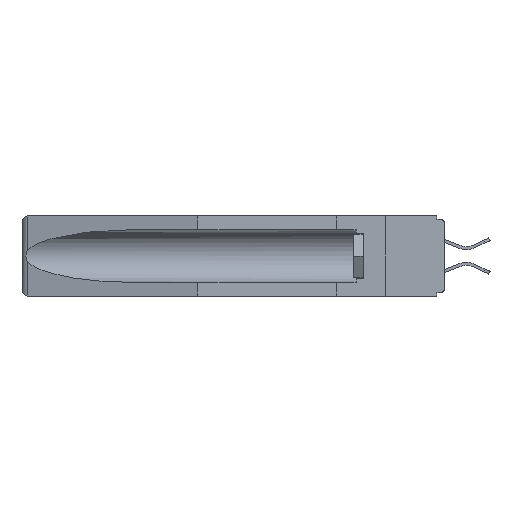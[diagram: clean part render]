
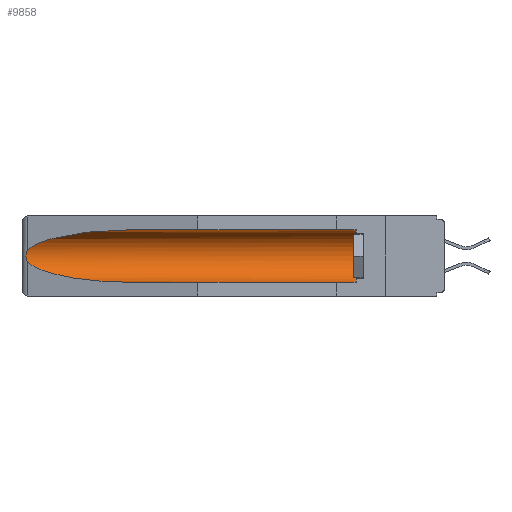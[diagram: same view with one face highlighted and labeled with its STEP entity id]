
A CAD part, left-side view. The second image highlights one B-rep face of the part: STEP entity #9858.
In plain terms, the highlighted cylindrical face has radius 2.857 mm (diameter 5.715 mm), a partial arc.
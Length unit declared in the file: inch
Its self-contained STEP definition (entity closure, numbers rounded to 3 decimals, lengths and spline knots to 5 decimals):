
#832 = CARTESIAN_POINT ( 'NONE',  ( 0.21114, 1.30732, -0.059 ) ) ;
#970 = EDGE_CURVE ( 'NONE', #17603, #32827, #12499, .T. ) ;
#3449 = VECTOR ( 'NONE', #21582, 39.37008 ) ;
#4038 = CARTESIAN_POINT ( 'NONE',  ( 0.2675, 1.53308, -0.16763 ) ) ;
#4170 = VERTEX_POINT ( 'NONE', #8145 ) ;
#4798 = CARTESIAN_POINT ( 'NONE',  ( 0.155, 1.07973, -0.059 ) ) ;
#6638 = ORIENTED_EDGE ( 'NONE', *, *, #20950, .T. ) ;
#6964 = FACE_OUTER_BOUND ( 'NONE', #16419, .T. ) ;
#7019 = CARTESIAN_POINT ( 'NONE',  ( 0.2673, 1.5327, -0.16383 ) ) ;
#7035 = CARTESIAN_POINT ( 'NONE',  ( 0.155, -0.30754, -0.284 ) ) ;
#7382 = CIRCLE ( 'NONE', #21650, 0.1125 ) ;
#7464 = CARTESIAN_POINT ( 'NONE',  ( 0.25451, 1.48313, -0.24835 ) ) ;
#7613 = ORIENTED_EDGE ( 'NONE', *, *, #23515, .T. ) ;
#8114 = DIRECTION ( 'NONE',  ( 0., 1., 0. ) ) ;
#8145 = CARTESIAN_POINT ( 'NONE',  ( 0.26537, 1.52718, -0.14972 ) ) ;
#8157 = ORIENTED_EDGE ( 'NONE', *, *, #33578, .T. ) ;
#8861 = VERTEX_POINT ( 'NONE', #4798 ) ;
#9524 = CARTESIAN_POINT ( 'NONE',  ( 0.26537, 1.52718, -0.14972 ) ) ;
#9638 = CARTESIAN_POINT ( 'NONE',  ( 0.2673, 1.53269, -0.17917 ) ) ;
#9858 = ADVANCED_FACE ( 'NONE', ( #6964 ), #26909, .F. ) ;
#10532 = DIRECTION ( 'NONE',  ( 0., 0., 1. ) ) ;
#10915 = VERTEX_POINT ( 'NONE', #13746 ) ;
#10970 = CARTESIAN_POINT ( 'NONE',  ( 0.155, 0.126, -0.1715 ) ) ;
#11829 = CARTESIAN_POINT ( 'NONE',  ( 0.26537, 1.52718, -0.19328 ) ) ;
#12499 = LINE ( 'NONE', #7035, #28349 ) ;
#12506 = CARTESIAN_POINT ( 'NONE',  ( 0.155, 1.07973, -0.284 ) ) ;
#13746 = CARTESIAN_POINT ( 'NONE',  ( 0.155, 0.126, -0.059 ) ) ;
#13822 = DIRECTION ( 'NONE',  ( 0., -1., 0. ) ) ;
#14091 = CARTESIAN_POINT ( 'NONE',  ( 0.155, 0.126, -0.284 ) ) ;
#14318 = AXIS2_PLACEMENT_3D ( 'NONE', #20671, #8114, #10532 ) ;
#16350 = CARTESIAN_POINT ( 'NONE',  ( 0.26537, 1.52718, -0.19328 ) ) ;
#16419 = EDGE_LOOP ( 'NONE', ( #7613, #6638, #19273, #22211, #30558, #8157 ) ) ;
#17603 = VERTEX_POINT ( 'NONE', #14091 ) ;
#17896 = EDGE_CURVE ( 'NONE', #17603, #10915, #7382, .T. ) ;
#17945 = CARTESIAN_POINT ( 'NONE',  ( 0.21114, 1.30732, -0.284 ) ) ;
#18059 =( BOUNDED_CURVE ( )  B_SPLINE_CURVE ( 3, ( #24129, #832, #24013, #18816 ),
 .UNSPECIFIED., .F., .F. ) 
 B_SPLINE_CURVE_WITH_KNOTS ( ( 4, 4 ),
 ( 4.71239, 6.08839 ),
 .UNSPECIFIED. ) 
 CURVE ( )  GEOMETRIC_REPRESENTATION_ITEM ( )  RATIONAL_B_SPLINE_CURVE ( ( 1., 0.848, 0.848, 1. ) ) 
 REPRESENTATION_ITEM ( '' )  );
#18816 = CARTESIAN_POINT ( 'NONE',  ( 0.26537, 1.52718, -0.14972 ) ) ;
#19108 = CARTESIAN_POINT ( 'NONE',  ( 0.155, 1.07973, -0.284 ) ) ;
#19273 = ORIENTED_EDGE ( 'NONE', *, *, #23360, .T. ) ;
#20671 = CARTESIAN_POINT ( 'NONE',  ( 0.155, -0.30754, -0.1715 ) ) ;
#20950 = EDGE_CURVE ( 'NONE', #4170, #21561, #26594, .T. ) ;
#21013 = LINE ( 'NONE', #32392, #3449 ) ;
#21561 = VERTEX_POINT ( 'NONE', #16350 ) ;
#21582 = DIRECTION ( 'NONE',  ( 0., 1., 0. ) ) ;
#21650 = AXIS2_PLACEMENT_3D ( 'NONE', #10970, #13822, #31979 ) ;
#22211 = ORIENTED_EDGE ( 'NONE', *, *, #970, .F. ) ;
#22251 = CARTESIAN_POINT ( 'NONE',  ( 0.26655, 1.53094, -0.18657 ) ) ;
#22564 = CARTESIAN_POINT ( 'NONE',  ( 0.26654, 1.53092, -0.15636 ) ) ;
#23360 = EDGE_CURVE ( 'NONE', #21561, #32827, #27018, .T. ) ;
#23515 = EDGE_CURVE ( 'NONE', #8861, #4170, #18059, .T. ) ;
#24013 = CARTESIAN_POINT ( 'NONE',  ( 0.25451, 1.48313, -0.09465 ) ) ;
#24129 = CARTESIAN_POINT ( 'NONE',  ( 0.155, 1.07973, -0.059 ) ) ;
#25230 = CARTESIAN_POINT ( 'NONE',  ( 0.2675, 1.53308, -0.17534 ) ) ;
#26594 = B_SPLINE_CURVE_WITH_KNOTS ( 'NONE', 3,
 ( #9524, #32739, #22564, #7019, #4038, #25230, #9638, #22251, #27404, #11829 ),
 .UNSPECIFIED., .F., .F.,
 ( 4, 2, 2, 2, 4 ),
 ( 0., 0.00029, 0.00058, 0.00087, 0.00117 ),
 .UNSPECIFIED. ) ;
#26909 = CYLINDRICAL_SURFACE ( 'NONE', #14318, 0.1125 ) ;
#27018 =( BOUNDED_CURVE ( )  B_SPLINE_CURVE ( 3, ( #33539, #7464, #17945, #12506 ),
 .UNSPECIFIED., .F., .F. ) 
 B_SPLINE_CURVE_WITH_KNOTS ( ( 4, 4 ),
 ( 0.1948, 1.5708 ),
 .UNSPECIFIED. ) 
 CURVE ( )  GEOMETRIC_REPRESENTATION_ITEM ( )  RATIONAL_B_SPLINE_CURVE ( ( 1., 0.848, 0.848, 1. ) ) 
 REPRESENTATION_ITEM ( '' )  );
#27404 = CARTESIAN_POINT ( 'NONE',  ( 0.26597, 1.5296, -0.19026 ) ) ;
#28349 = VECTOR ( 'NONE', #32529, 39.37008 ) ;
#30558 = ORIENTED_EDGE ( 'NONE', *, *, #17896, .T. ) ;
#31979 = DIRECTION ( 'NONE',  ( 0., 0., 1. ) ) ;
#32392 = CARTESIAN_POINT ( 'NONE',  ( 0.155, -0.30754, -0.059 ) ) ;
#32529 = DIRECTION ( 'NONE',  ( 0., 1., 0. ) ) ;
#32739 = CARTESIAN_POINT ( 'NONE',  ( 0.26597, 1.52961, -0.15275 ) ) ;
#32827 = VERTEX_POINT ( 'NONE', #19108 ) ;
#33539 = CARTESIAN_POINT ( 'NONE',  ( 0.26537, 1.52718, -0.19328 ) ) ;
#33578 = EDGE_CURVE ( 'NONE', #10915, #8861, #21013, .T. ) ;
